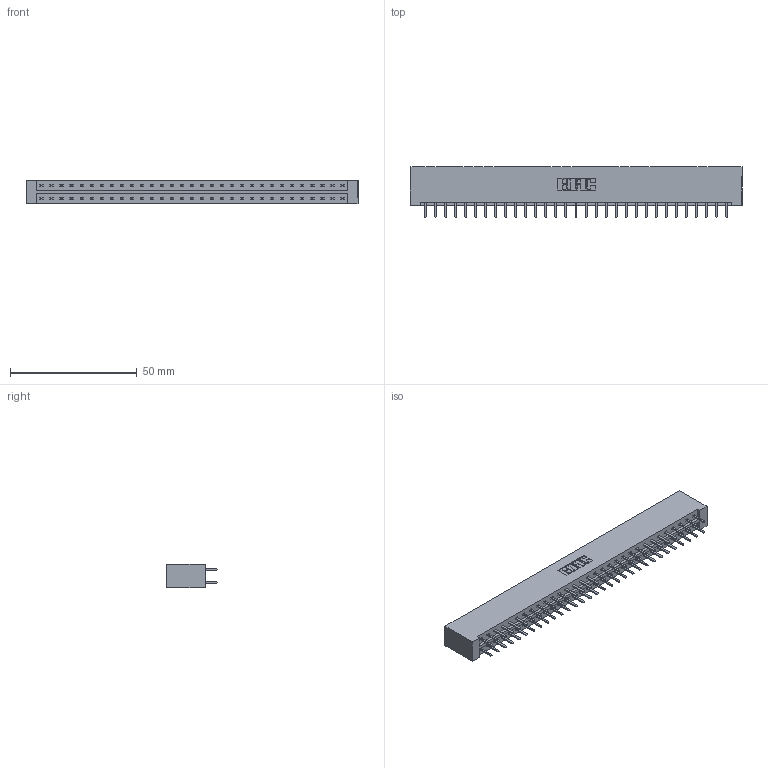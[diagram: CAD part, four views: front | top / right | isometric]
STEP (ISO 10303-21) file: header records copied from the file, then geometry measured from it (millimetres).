
FILE_DESCRIPTION (( 'STEP AP203' ), '1' );
FILE_NAME ('833-062-520-201.STEP', '2020-06-05T05:04:25', ( '' ), ( '' ), 'SwSTEP 2.0', 'SolidWorks 2020', '' );
FILE_SCHEMA (( 'CONFIG_CONTROL_DESIGN' ));
Length unit declared in the file: inch
Products named in the file (3): 833-062-520-201; 833 Part_Lugless; 345-292-001_345-293-120
Assembly tree (63 placements, depth 2):
  833-062-520-201
    833 Part_Lugless
    345-292-001_345-293-120  x62
Bounding box: 131.09 x 20.02 x 9.4 mm (x, y, z)
Volume: 13885.6 mm3; surface area: 16250.2 mm2
Topology: 63 solids, 63 shells, 3578 faces, 10393 edges, 6762 vertices
Faces by surface type: plane 2422, cylinder 1156
Entity records: 21203 total; most frequent: CARTESIAN_POINT 3538, ORIENTED_EDGE 3462, DIRECTION 3023, EDGE_CURVE 1731, LINE 1607, VECTOR 1607, VERTEX_POINT 1150, AXIS2_PLACEMENT_3D 708
